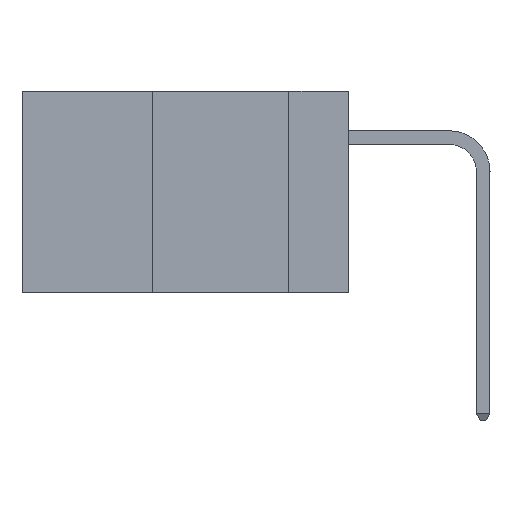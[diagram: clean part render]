
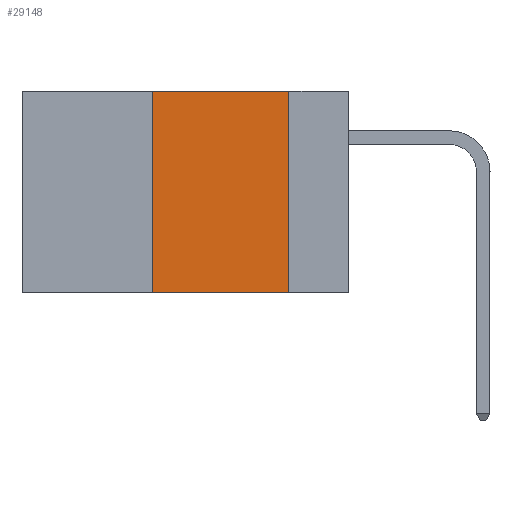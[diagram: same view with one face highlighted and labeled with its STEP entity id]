
A CAD part, left-side view. The second image highlights one B-rep face of the part: STEP entity #29148.
In plain terms, the highlighted planar face has unit normal (-1, 0, 0).
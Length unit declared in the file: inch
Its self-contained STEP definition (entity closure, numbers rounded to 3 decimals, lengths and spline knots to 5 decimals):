
#562 = CARTESIAN_POINT ( 'NONE',  ( 0., 0.6, 0. ) ) ;
#994 = CARTESIAN_POINT ( 'NONE',  ( 0., 0.11, 0. ) ) ;
#2256 = ORIENTED_EDGE ( 'NONE', *, *, #32519, .F. ) ;
#2692 = CARTESIAN_POINT ( 'NONE',  ( 0., 0.11, 0. ) ) ;
#4883 = ORIENTED_EDGE ( 'NONE', *, *, #14117, .F. ) ;
#5279 = CARTESIAN_POINT ( 'NONE',  ( 0., 0.36, 0. ) ) ;
#6096 = EDGE_LOOP ( 'NONE', ( #29607, #2256, #4883, #18301 ) ) ;
#6863 = VERTEX_POINT ( 'NONE', #41733 ) ;
#8214 = PLANE ( 'NONE',  #31660 ) ;
#9030 = CARTESIAN_POINT ( 'NONE',  ( 0., 0.6, -0.37 ) ) ;
#9751 = CARTESIAN_POINT ( 'NONE',  ( 0., 0.36, -0.37 ) ) ;
#11568 = DIRECTION ( 'NONE',  ( 0., 0., -1. ) ) ;
#11646 = VERTEX_POINT ( 'NONE', #9751 ) ;
#13429 = VECTOR ( 'NONE', #23715, 39.37008 ) ;
#14117 = EDGE_CURVE ( 'NONE', #11646, #6863, #42248, .T. ) ;
#14708 = VERTEX_POINT ( 'NONE', #18101 ) ;
#15258 = DIRECTION ( 'NONE',  ( 0., 0., 1. ) ) ;
#15297 = VECTOR ( 'NONE', #24143, 39.37008 ) ;
#15515 = EDGE_CURVE ( 'NONE', #11646, #14708, #37997, .T. ) ;
#18088 = CARTESIAN_POINT ( 'NONE',  ( 0., 0.6, 0. ) ) ;
#18101 = CARTESIAN_POINT ( 'NONE',  ( 0., 0.11, -0.37 ) ) ;
#18301 = ORIENTED_EDGE ( 'NONE', *, *, #15515, .T. ) ;
#23715 = DIRECTION ( 'NONE',  ( 0., -1., 0. ) ) ;
#24143 = DIRECTION ( 'NONE',  ( 0., 0., -1. ) ) ;
#24631 = VECTOR ( 'NONE', #15258, 39.37008 ) ;
#24921 = VERTEX_POINT ( 'NONE', #2692 ) ;
#29148 = ADVANCED_FACE ( 'NONE', ( #36985 ), #8214, .F. ) ;
#29607 = ORIENTED_EDGE ( 'NONE', *, *, #35685, .F. ) ;
#30185 = VECTOR ( 'NONE', #32205, 39.37008 ) ;
#31406 = DIRECTION ( 'NONE',  ( 1., 0., 0. ) ) ;
#31660 = AXIS2_PLACEMENT_3D ( 'NONE', #18088, #31406, #11568 ) ;
#32087 = LINE ( 'NONE', #562, #13429 ) ;
#32205 = DIRECTION ( 'NONE',  ( 0., -1., 0. ) ) ;
#32519 = EDGE_CURVE ( 'NONE', #6863, #24921, #32087, .T. ) ;
#33956 = LINE ( 'NONE', #994, #15297 ) ;
#35685 = EDGE_CURVE ( 'NONE', #24921, #14708, #33956, .T. ) ;
#36985 = FACE_OUTER_BOUND ( 'NONE', #6096, .T. ) ;
#37997 = LINE ( 'NONE', #9030, #30185 ) ;
#41733 = CARTESIAN_POINT ( 'NONE',  ( 0., 0.36, 0. ) ) ;
#42248 = LINE ( 'NONE', #5279, #24631 ) ;
